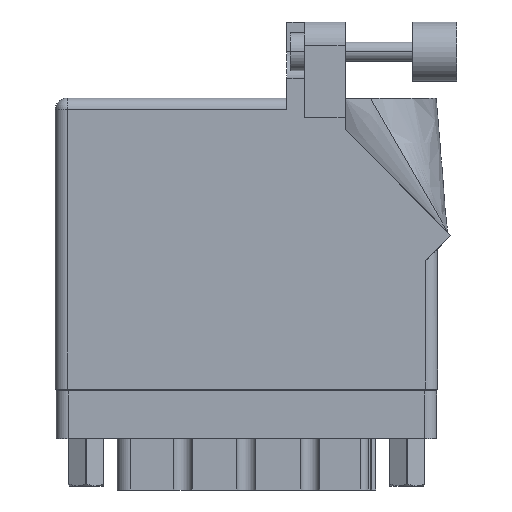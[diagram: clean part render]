
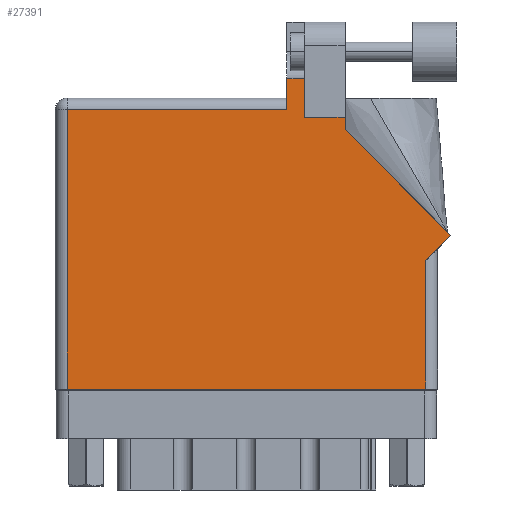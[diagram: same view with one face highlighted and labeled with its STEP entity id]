
A CAD part, front view. The second image highlights one B-rep face of the part: STEP entity #27391.
In plain terms, the highlighted face is planar.
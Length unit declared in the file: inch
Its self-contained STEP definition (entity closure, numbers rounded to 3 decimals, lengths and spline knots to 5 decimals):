
#297 = EDGE_CURVE ( 'NONE', #11770, #5305, #32065, .T. ) ;
#548 = CARTESIAN_POINT ( 'NONE',  ( 1.311, 1.43, 0. ) ) ;
#1379 = ORIENTED_EDGE ( 'NONE', *, *, #297, .T. ) ;
#1615 = DIRECTION ( 'NONE',  ( 0., -1., 0. ) ) ;
#2828 = ORIENTED_EDGE ( 'NONE', *, *, #42082, .T. ) ;
#2859 = DIRECTION ( 'NONE',  ( 0., 0., -1. ) ) ;
#2874 = DIRECTION ( 'NONE',  ( 0.707, 0.707, 0. ) ) ;
#2923 = ORIENTED_EDGE ( 'NONE', *, *, #13789, .T. ) ;
#3883 = DIRECTION ( 'NONE',  ( 0., 1., 0. ) ) ;
#3984 = FACE_OUTER_BOUND ( 'NONE', #33367, .T. ) ;
#4545 = CARTESIAN_POINT ( 'NONE',  ( 0., 1.468, 0. ) ) ;
#4702 = DIRECTION ( 'NONE',  ( -1., 0., 0. ) ) ;
#4947 = LINE ( 'NONE', #30281, #8310 ) ;
#5305 = VERTEX_POINT ( 'NONE', #37062 ) ;
#5906 = EDGE_CURVE ( 'NONE', #22767, #20705, #32720, .T. ) ;
#6533 = EDGE_CURVE ( 'NONE', #31037, #11770, #44399, .T. ) ;
#8310 = VECTOR ( 'NONE', #24031, 39.37008 ) ;
#8443 = LINE ( 'NONE', #45267, #34808 ) ;
#9449 = VECTOR ( 'NONE', #18901, 39.37008 ) ;
#9611 = DIRECTION ( 'NONE',  ( -1., 0., 0. ) ) ;
#9661 = ORIENTED_EDGE ( 'NONE', *, *, #6533, .T. ) ;
#10162 = CARTESIAN_POINT ( 'NONE',  ( 1.311, 1.6315, 0. ) ) ;
#10385 = CARTESIAN_POINT ( 'NONE',  ( 0.062, 1.468, 0. ) ) ;
#10767 = CARTESIAN_POINT ( 'NONE',  ( 1.524, 1.36442, 0. ) ) ;
#11770 = VERTEX_POINT ( 'NONE', #21173 ) ;
#13100 = CARTESIAN_POINT ( 'NONE',  ( 1.948, 0.737, 0. ) ) ;
#13592 = VECTOR ( 'NONE', #2874, 39.37008 ) ;
#13789 = EDGE_CURVE ( 'NONE', #18842, #24478, #8443, .T. ) ;
#15388 = EDGE_CURVE ( 'NONE', #29808, #18842, #26682, .T. ) ;
#15917 = CARTESIAN_POINT ( 'NONE',  ( 0.062, 0., 0. ) ) ;
#16428 = CARTESIAN_POINT ( 'NONE',  ( 1.217, 1.53, 0. ) ) ;
#16438 = ORIENTED_EDGE ( 'NONE', *, *, #5906, .T. ) ;
#17270 = CARTESIAN_POINT ( 'NONE',  ( 1.948, 0., 0. ) ) ;
#17614 = CARTESIAN_POINT ( 'NONE',  ( 1.217, 1.468, 0. ) ) ;
#17706 = VECTOR ( 'NONE', #27357, 39.37008 ) ;
#18790 = LINE ( 'NONE', #16428, #33950 ) ;
#18842 = VERTEX_POINT ( 'NONE', #10162 ) ;
#18901 = DIRECTION ( 'NONE',  ( 1., 0., 0. ) ) ;
#18972 = EDGE_CURVE ( 'NONE', #28717, #26586, #30030, .T. ) ;
#19114 = ORIENTED_EDGE ( 'NONE', *, *, #43597, .T. ) ;
#20006 = CARTESIAN_POINT ( 'NONE',  ( 1.524, 1.43, 0. ) ) ;
#20199 = DIRECTION ( 'NONE',  ( 0., -1., 0. ) ) ;
#20318 = CARTESIAN_POINT ( 'NONE',  ( 1.311, 1.43, 0. ) ) ;
#20705 = VERTEX_POINT ( 'NONE', #15917 ) ;
#21173 = CARTESIAN_POINT ( 'NONE',  ( 1.948, 0.675, 0. ) ) ;
#21653 = ORIENTED_EDGE ( 'NONE', *, *, #15388, .T. ) ;
#22767 = VERTEX_POINT ( 'NONE', #10385 ) ;
#23233 = ORIENTED_EDGE ( 'NONE', *, *, #18972, .T. ) ;
#23529 = CARTESIAN_POINT ( 'NONE',  ( 0.062, 0., 0. ) ) ;
#24031 = DIRECTION ( 'NONE',  ( -0.707, 0.707, 0. ) ) ;
#24478 = VERTEX_POINT ( 'NONE', #32646 ) ;
#24626 = CARTESIAN_POINT ( 'NONE',  ( 0., 1.53, 0. ) ) ;
#25608 = DIRECTION ( 'NONE',  ( 0., 1., 0. ) ) ;
#26108 = VECTOR ( 'NONE', #4702, 39.37008 ) ;
#26586 = VERTEX_POINT ( 'NONE', #40619 ) ;
#26682 = LINE ( 'NONE', #548, #38963 ) ;
#26718 = EDGE_CURVE ( 'NONE', #20705, #31037, #37430, .T. ) ;
#27357 = DIRECTION ( 'NONE',  ( -1., 0., 0. ) ) ;
#27369 = DIRECTION ( 'NONE',  ( 0., 1., 0. ) ) ;
#27391 = ADVANCED_FACE ( 'NONE', ( #3984 ), #28075, .F. ) ;
#28035 = ORIENTED_EDGE ( 'NONE', *, *, #31362, .T. ) ;
#28075 = PLANE ( 'NONE',  #31474 ) ;
#28717 = VERTEX_POINT ( 'NONE', #32026 ) ;
#28888 = LINE ( 'NONE', #20006, #17706 ) ;
#29808 = VERTEX_POINT ( 'NONE', #20318 ) ;
#30030 = LINE ( 'NONE', #10767, #33449 ) ;
#30281 = CARTESIAN_POINT ( 'NONE',  ( 2.08071, 0.80771, 0. ) ) ;
#30898 = EDGE_CURVE ( 'NONE', #36855, #22767, #31736, .T. ) ;
#31037 = VERTEX_POINT ( 'NONE', #17270 ) ;
#31362 = EDGE_CURVE ( 'NONE', #24478, #36855, #18790, .T. ) ;
#31474 = AXIS2_PLACEMENT_3D ( 'NONE', #24626, #2859, #45402 ) ;
#31736 = LINE ( 'NONE', #4545, #26108 ) ;
#32026 = CARTESIAN_POINT ( 'NONE',  ( 1.524, 1.36442, 0. ) ) ;
#32065 = LINE ( 'NONE', #46206, #13592 ) ;
#32646 = CARTESIAN_POINT ( 'NONE',  ( 1.217, 1.6315, 0. ) ) ;
#32720 = LINE ( 'NONE', #23529, #39416 ) ;
#33367 = EDGE_LOOP ( 'NONE', ( #21653, #2923, #28035, #41900, #16438, #37663, #9661, #1379, #2828, #23233, #19114 ) ) ;
#33449 = VECTOR ( 'NONE', #3883, 39.37008 ) ;
#33950 = VECTOR ( 'NONE', #20199, 39.37008 ) ;
#34808 = VECTOR ( 'NONE', #9611, 39.37008 ) ;
#36855 = VERTEX_POINT ( 'NONE', #17614 ) ;
#36887 = CARTESIAN_POINT ( 'NONE',  ( 0., 0., 0. ) ) ;
#37062 = CARTESIAN_POINT ( 'NONE',  ( 2.08071, 0.80771, 0. ) ) ;
#37430 = LINE ( 'NONE', #36887, #9449 ) ;
#37663 = ORIENTED_EDGE ( 'NONE', *, *, #26718, .T. ) ;
#38963 = VECTOR ( 'NONE', #25608, 39.37008 ) ;
#39416 = VECTOR ( 'NONE', #1615, 39.37008 ) ;
#40619 = CARTESIAN_POINT ( 'NONE',  ( 1.524, 1.43, 0. ) ) ;
#41900 = ORIENTED_EDGE ( 'NONE', *, *, #30898, .T. ) ;
#42082 = EDGE_CURVE ( 'NONE', #5305, #28717, #4947, .T. ) ;
#43597 = EDGE_CURVE ( 'NONE', #26586, #29808, #28888, .T. ) ;
#44399 = LINE ( 'NONE', #13100, #46084 ) ;
#45267 = CARTESIAN_POINT ( 'NONE',  ( 1.64177, 1.6315, 0. ) ) ;
#45402 = DIRECTION ( 'NONE',  ( -1., 0., 0. ) ) ;
#46084 = VECTOR ( 'NONE', #27369, 39.37008 ) ;
#46206 = CARTESIAN_POINT ( 'NONE',  ( 2.01, 0.737, 0. ) ) ;
